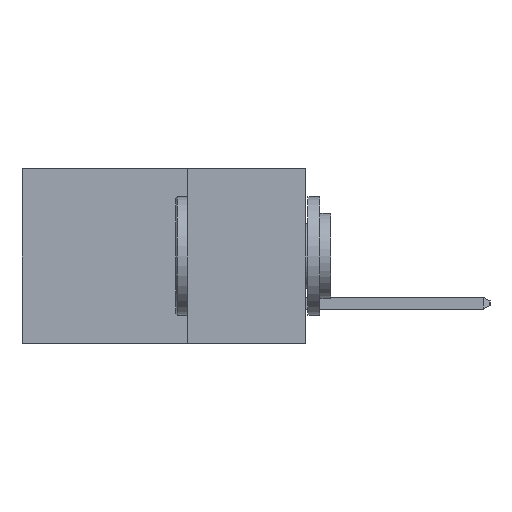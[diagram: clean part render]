
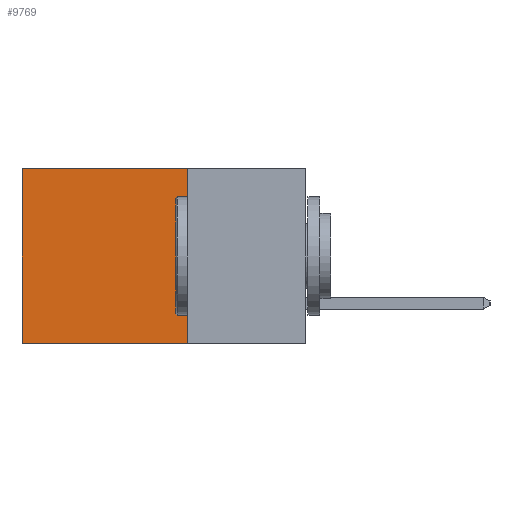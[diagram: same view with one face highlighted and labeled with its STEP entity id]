
A CAD part, left-side view. The second image highlights one B-rep face of the part: STEP entity #9769.
In plain terms, the highlighted planar face has unit normal (-1, 0, 0).
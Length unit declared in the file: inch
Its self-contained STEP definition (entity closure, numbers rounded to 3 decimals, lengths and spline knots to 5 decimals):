
#112 = EDGE_CURVE ( 'NONE', #12210, #11387, #6494, .T. ) ;
#287 = DIRECTION ( 'NONE',  ( 0., 0., -1. ) ) ;
#1562 = VECTOR ( 'NONE', #12030, 39.37008 ) ;
#2028 = CARTESIAN_POINT ( 'NONE',  ( 0.2615, 0.6, -0.37 ) ) ;
#2169 = VERTEX_POINT ( 'NONE', #2028 ) ;
#3346 = VERTEX_POINT ( 'NONE', #12482 ) ;
#3638 = DIRECTION ( 'NONE',  ( 0., 0., -1. ) ) ;
#4088 = LINE ( 'NONE', #5558, #11022 ) ;
#4225 = VECTOR ( 'NONE', #3638, 39.37008 ) ;
#4270 = CARTESIAN_POINT ( 'NONE',  ( 0.2615, 0.25, -0.37 ) ) ;
#5124 = FACE_OUTER_BOUND ( 'NONE', #12690, .T. ) ;
#5546 = LINE ( 'NONE', #4270, #1562 ) ;
#5558 = CARTESIAN_POINT ( 'NONE',  ( 0.2615, 0.25, 0. ) ) ;
#6255 = CARTESIAN_POINT ( 'NONE',  ( 0.2615, 0.6, -0.37 ) ) ;
#6447 = CARTESIAN_POINT ( 'NONE',  ( 0.2615, 0.25, 0. ) ) ;
#6494 = LINE ( 'NONE', #14759, #10388 ) ;
#6848 = DIRECTION ( 'NONE',  ( 0., 1., 0. ) ) ;
#6916 = PLANE ( 'NONE',  #13167 ) ;
#8250 = DIRECTION ( 'NONE',  ( 1., 0., 0. ) ) ;
#8472 = EDGE_CURVE ( 'NONE', #12210, #3346, #4088, .T. ) ;
#9765 = EDGE_CURVE ( 'NONE', #11387, #2169, #5546, .T. ) ;
#9769 = ADVANCED_FACE ( 'NONE', ( #5124 ), #6916, .F. ) ;
#10100 = ORIENTED_EDGE ( 'NONE', *, *, #9765, .F. ) ;
#10388 = VECTOR ( 'NONE', #15296, 39.37008 ) ;
#11022 = VECTOR ( 'NONE', #6848, 39.37008 ) ;
#11155 = LINE ( 'NONE', #6255, #4225 ) ;
#11387 = VERTEX_POINT ( 'NONE', #13855 ) ;
#12030 = DIRECTION ( 'NONE',  ( 0., 1., 0. ) ) ;
#12210 = VERTEX_POINT ( 'NONE', #6447 ) ;
#12482 = CARTESIAN_POINT ( 'NONE',  ( 0.2615, 0.6, 0. ) ) ;
#12502 = ORIENTED_EDGE ( 'NONE', *, *, #112, .F. ) ;
#12690 = EDGE_LOOP ( 'NONE', ( #16652, #10100, #12502, #13838 ) ) ;
#13167 = AXIS2_PLACEMENT_3D ( 'NONE', #15755, #8250, #287 ) ;
#13838 = ORIENTED_EDGE ( 'NONE', *, *, #8472, .T. ) ;
#13855 = CARTESIAN_POINT ( 'NONE',  ( 0.2615, 0.25, -0.37 ) ) ;
#14759 = CARTESIAN_POINT ( 'NONE',  ( 0.2615, 0.25, -0.37 ) ) ;
#14879 = EDGE_CURVE ( 'NONE', #3346, #2169, #11155, .T. ) ;
#15296 = DIRECTION ( 'NONE',  ( 0., 0., -1. ) ) ;
#15755 = CARTESIAN_POINT ( 'NONE',  ( 0.2615, 0.25, -0.37 ) ) ;
#16652 = ORIENTED_EDGE ( 'NONE', *, *, #14879, .T. ) ;
